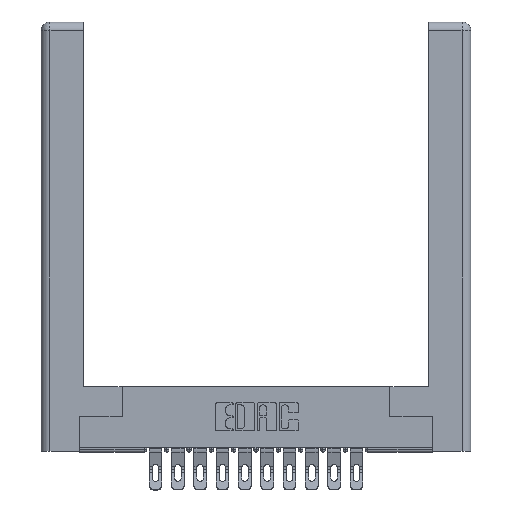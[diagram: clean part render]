
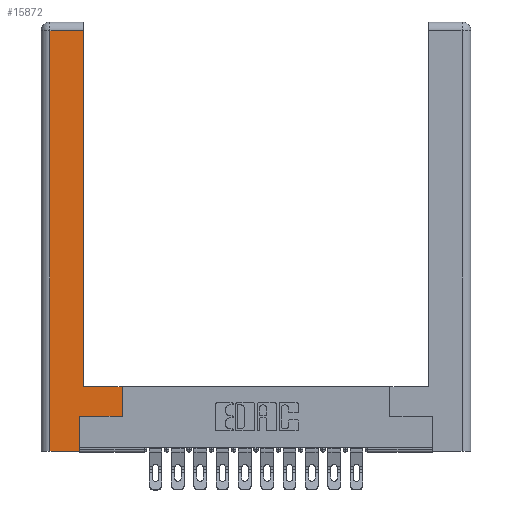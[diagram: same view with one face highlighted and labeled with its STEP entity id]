
A CAD part, top view. The second image highlights one B-rep face of the part: STEP entity #15872.
In plain terms, the highlighted planar face has unit normal (0, 0, 1).
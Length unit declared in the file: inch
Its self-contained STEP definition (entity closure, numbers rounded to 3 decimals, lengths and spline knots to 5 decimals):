
#78 = CARTESIAN_POINT ( 'NONE',  ( 0.0615, 2.94, 0. ) ) ;
#164 = ORIENTED_EDGE ( 'NONE', *, *, #3041, .T. ) ;
#174 = DIRECTION ( 'NONE',  ( -1., 0., 0. ) ) ;
#228 = CARTESIAN_POINT ( 'NONE',  ( 0.0615, 2.94, 0. ) ) ;
#482 = CARTESIAN_POINT ( 'NONE',  ( 0.265, 0., 0. ) ) ;
#964 = VECTOR ( 'NONE', #3173, 39.37008 ) ;
#1025 = VERTEX_POINT ( 'NONE', #3296 ) ;
#1171 = CARTESIAN_POINT ( 'NONE',  ( 0.295, 0.45, 0. ) ) ;
#1441 = CARTESIAN_POINT ( 'NONE',  ( 0.295, 0.45, 0. ) ) ;
#2726 = CARTESIAN_POINT ( 'NONE',  ( 0.565, 0.45, 0. ) ) ;
#3041 = EDGE_CURVE ( 'NONE', #7280, #14806, #13969, .T. ) ;
#3173 = DIRECTION ( 'NONE',  ( 1., 0., 0. ) ) ;
#3296 = CARTESIAN_POINT ( 'NONE',  ( 0.265, 0., 0. ) ) ;
#3540 = CARTESIAN_POINT ( 'NONE',  ( 0.0615, 0., 0. ) ) ;
#3888 = ORIENTED_EDGE ( 'NONE', *, *, #7037, .T. ) ;
#4152 = CARTESIAN_POINT ( 'NONE',  ( 0., 0., 0. ) ) ;
#4593 = CARTESIAN_POINT ( 'NONE',  ( 0.295, 2.94, 0. ) ) ;
#4801 = CARTESIAN_POINT ( 'NONE',  ( 0.565, 0.245, 0. ) ) ;
#4865 = ORIENTED_EDGE ( 'NONE', *, *, #12969, .T. ) ;
#5086 = EDGE_CURVE ( 'NONE', #17978, #16801, #9570, .T. ) ;
#5270 = EDGE_LOOP ( 'NONE', ( #9030, #11742, #164, #8656, #3888, #4865, #14046, #10488 ) ) ;
#5823 = VECTOR ( 'NONE', #17992, 39.37008 ) ;
#6100 = CARTESIAN_POINT ( 'NONE',  ( 0.295, 3., 0. ) ) ;
#6928 = PLANE ( 'NONE',  #12216 ) ;
#7037 = EDGE_CURVE ( 'NONE', #1025, #13663, #9294, .T. ) ;
#7130 = LINE ( 'NONE', #1441, #5823 ) ;
#7280 = VERTEX_POINT ( 'NONE', #78 ) ;
#7755 = CARTESIAN_POINT ( 'NONE',  ( 0.565, 0.245, 0. ) ) ;
#8333 = FACE_OUTER_BOUND ( 'NONE', #5270, .T. ) ;
#8383 = EDGE_CURVE ( 'NONE', #14785, #9527, #11025, .T. ) ;
#8416 = CARTESIAN_POINT ( 'NONE',  ( 0.265, 0.245, 0. ) ) ;
#8552 = LINE ( 'NONE', #482, #964 ) ;
#8656 = ORIENTED_EDGE ( 'NONE', *, *, #15982, .T. ) ;
#9030 = ORIENTED_EDGE ( 'NONE', *, *, #5086, .T. ) ;
#9068 = VECTOR ( 'NONE', #14872, 39.37008 ) ;
#9294 = LINE ( 'NONE', #8416, #17807 ) ;
#9527 = VERTEX_POINT ( 'NONE', #13616 ) ;
#9570 = LINE ( 'NONE', #6100, #16559 ) ;
#10231 = VECTOR ( 'NONE', #12094, 39.37008 ) ;
#10488 = ORIENTED_EDGE ( 'NONE', *, *, #11993, .T. ) ;
#11025 = LINE ( 'NONE', #2726, #15165 ) ;
#11742 = ORIENTED_EDGE ( 'NONE', *, *, #12444, .T. ) ;
#11993 = EDGE_CURVE ( 'NONE', #9527, #17978, #7130, .T. ) ;
#12094 = DIRECTION ( 'NONE',  ( 0., -1., 0. ) ) ;
#12216 = AXIS2_PLACEMENT_3D ( 'NONE', #4152, #16834, #15324 ) ;
#12444 = EDGE_CURVE ( 'NONE', #16801, #7280, #12623, .T. ) ;
#12535 = CARTESIAN_POINT ( 'NONE',  ( 0.265, 0.245, 0. ) ) ;
#12538 = DIRECTION ( 'NONE',  ( 0., 1., 0. ) ) ;
#12623 = LINE ( 'NONE', #228, #15441 ) ;
#12969 = EDGE_CURVE ( 'NONE', #13663, #14785, #15205, .T. ) ;
#13217 = DIRECTION ( 'NONE',  ( 0., 1., 0. ) ) ;
#13616 = CARTESIAN_POINT ( 'NONE',  ( 0.565, 0.45, 0. ) ) ;
#13663 = VERTEX_POINT ( 'NONE', #12535 ) ;
#13969 = LINE ( 'NONE', #17434, #10231 ) ;
#14046 = ORIENTED_EDGE ( 'NONE', *, *, #8383, .T. ) ;
#14785 = VERTEX_POINT ( 'NONE', #4801 ) ;
#14806 = VERTEX_POINT ( 'NONE', #3540 ) ;
#14872 = DIRECTION ( 'NONE',  ( 1., 0., 0. ) ) ;
#15165 = VECTOR ( 'NONE', #12538, 39.37008 ) ;
#15205 = LINE ( 'NONE', #7755, #9068 ) ;
#15324 = DIRECTION ( 'NONE',  ( -1., 0., 0. ) ) ;
#15441 = VECTOR ( 'NONE', #174, 39.37008 ) ;
#15872 = ADVANCED_FACE ( 'NONE', ( #8333 ), #6928, .F. ) ;
#15982 = EDGE_CURVE ( 'NONE', #14806, #1025, #8552, .T. ) ;
#16559 = VECTOR ( 'NONE', #13217, 39.37008 ) ;
#16618 = DIRECTION ( 'NONE',  ( 0., 1., 0. ) ) ;
#16801 = VERTEX_POINT ( 'NONE', #4593 ) ;
#16834 = DIRECTION ( 'NONE',  ( 0., 0., -1. ) ) ;
#17434 = CARTESIAN_POINT ( 'NONE',  ( 0.0615, 0., 0. ) ) ;
#17807 = VECTOR ( 'NONE', #16618, 39.37008 ) ;
#17978 = VERTEX_POINT ( 'NONE', #1171 ) ;
#17992 = DIRECTION ( 'NONE',  ( -1., 0., 0. ) ) ;
